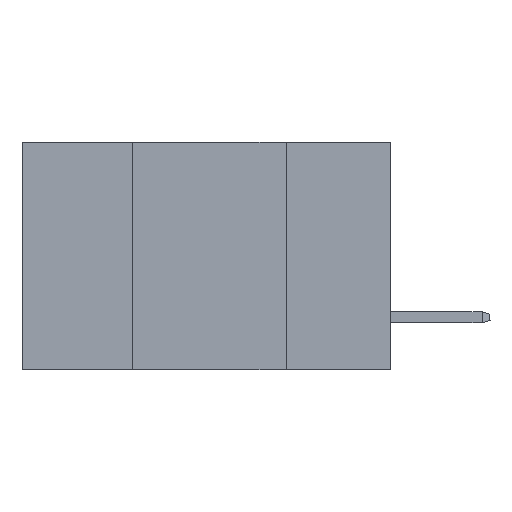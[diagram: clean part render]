
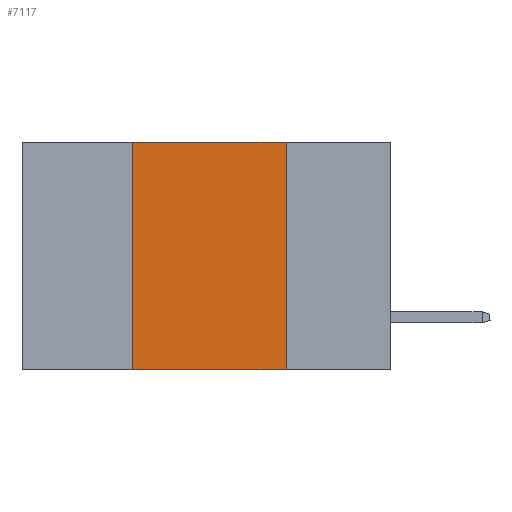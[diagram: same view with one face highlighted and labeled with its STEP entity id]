
A CAD part, left-side view. The second image highlights one B-rep face of the part: STEP entity #7117.
In plain terms, the highlighted planar face has unit normal (-1, 0, 0).
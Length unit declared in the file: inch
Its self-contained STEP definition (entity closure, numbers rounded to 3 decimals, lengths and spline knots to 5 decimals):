
#297 = DIRECTION ( 'NONE',  ( 0., 0., -1. ) ) ;
#968 = VECTOR ( 'NONE', #2664, 39.37008 ) ;
#1232 = LINE ( 'NONE', #10380, #5396 ) ;
#1261 = CARTESIAN_POINT ( 'NONE',  ( 0., 0.42, 0. ) ) ;
#1945 = VERTEX_POINT ( 'NONE', #8259 ) ;
#2552 = CARTESIAN_POINT ( 'NONE',  ( 0., 0.6, 0. ) ) ;
#2651 = EDGE_CURVE ( 'NONE', #4208, #1945, #8357, .T. ) ;
#2664 = DIRECTION ( 'NONE',  ( 0., -1., 0. ) ) ;
#2825 = VERTEX_POINT ( 'NONE', #8631 ) ;
#2960 = DIRECTION ( 'NONE',  ( 0., 0., 1. ) ) ;
#2993 = LINE ( 'NONE', #2552, #4931 ) ;
#3032 = ORIENTED_EDGE ( 'NONE', *, *, #9448, .F. ) ;
#4208 = VERTEX_POINT ( 'NONE', #8669 ) ;
#4512 = ORIENTED_EDGE ( 'NONE', *, *, #9893, .F. ) ;
#4631 = EDGE_CURVE ( 'NONE', #2825, #9169, #2993, .T. ) ;
#4882 = AXIS2_PLACEMENT_3D ( 'NONE', #9120, #9204, #4964 ) ;
#4931 = VECTOR ( 'NONE', #5780, 39.37008 ) ;
#4964 = DIRECTION ( 'NONE',  ( 0., 0., -1. ) ) ;
#5396 = VECTOR ( 'NONE', #297, 39.37008 ) ;
#5480 = ORIENTED_EDGE ( 'NONE', *, *, #2651, .T. ) ;
#5780 = DIRECTION ( 'NONE',  ( 0., -1., 0. ) ) ;
#6213 = ORIENTED_EDGE ( 'NONE', *, *, #4631, .F. ) ;
#6649 = EDGE_LOOP ( 'NONE', ( #4512, #6213, #3032, #5480 ) ) ;
#6878 = CARTESIAN_POINT ( 'NONE',  ( 0., 0.6, -0.37 ) ) ;
#7117 = ADVANCED_FACE ( 'NONE', ( #7773 ), #9965, .F. ) ;
#7773 = FACE_OUTER_BOUND ( 'NONE', #6649, .T. ) ;
#8259 = CARTESIAN_POINT ( 'NONE',  ( 0., 0.17, -0.37 ) ) ;
#8357 = LINE ( 'NONE', #6878, #968 ) ;
#8358 = VECTOR ( 'NONE', #2960, 39.37008 ) ;
#8564 = CARTESIAN_POINT ( 'NONE',  ( 0., 0.17, 0. ) ) ;
#8631 = CARTESIAN_POINT ( 'NONE',  ( 0., 0.42, 0. ) ) ;
#8669 = CARTESIAN_POINT ( 'NONE',  ( 0., 0.42, -0.37 ) ) ;
#9120 = CARTESIAN_POINT ( 'NONE',  ( 0., 0.6, 0. ) ) ;
#9169 = VERTEX_POINT ( 'NONE', #8564 ) ;
#9204 = DIRECTION ( 'NONE',  ( 1., 0., 0. ) ) ;
#9448 = EDGE_CURVE ( 'NONE', #4208, #2825, #9719, .T. ) ;
#9719 = LINE ( 'NONE', #1261, #8358 ) ;
#9893 = EDGE_CURVE ( 'NONE', #9169, #1945, #1232, .T. ) ;
#9965 = PLANE ( 'NONE',  #4882 ) ;
#10380 = CARTESIAN_POINT ( 'NONE',  ( 0., 0.17, 0. ) ) ;
